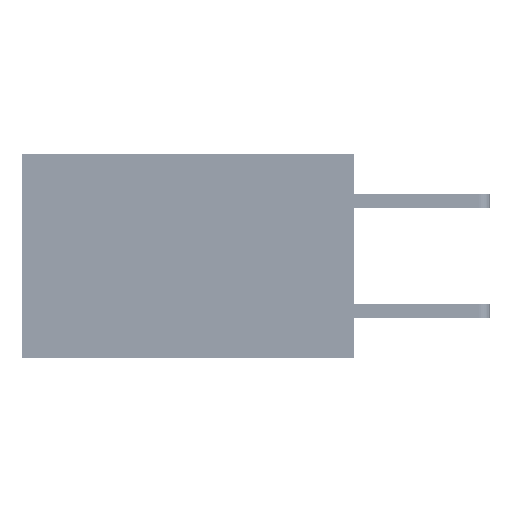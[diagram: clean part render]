
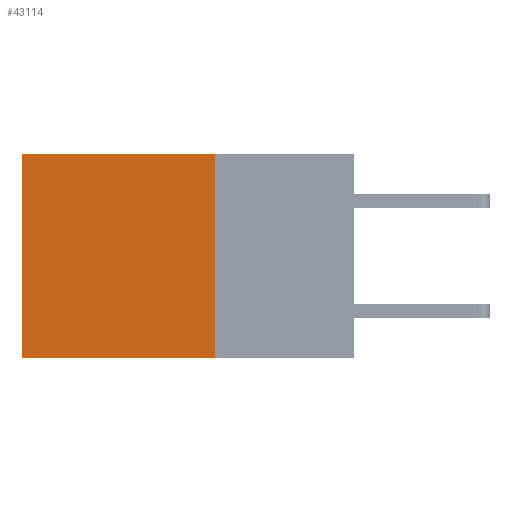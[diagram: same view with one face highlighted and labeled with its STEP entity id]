
A CAD part, left-side view. The second image highlights one B-rep face of the part: STEP entity #43114.
In plain terms, the highlighted planar face has unit normal (-1, 0, 0).
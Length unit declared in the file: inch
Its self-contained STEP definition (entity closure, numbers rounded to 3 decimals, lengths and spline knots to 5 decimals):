
#707 = DIRECTION ( 'NONE',  ( 0., 1., 0. ) ) ;
#711 = FACE_OUTER_BOUND ( 'NONE', #18224, .T. ) ;
#1418 = VERTEX_POINT ( 'NONE', #12976 ) ;
#2862 = LINE ( 'NONE', #3760, #28145 ) ;
#3760 = CARTESIAN_POINT ( 'NONE',  ( 0.2875, 0.6, 0. ) ) ;
#3798 = VERTEX_POINT ( 'NONE', #29327 ) ;
#6840 = LINE ( 'NONE', #11365, #21431 ) ;
#9747 = VECTOR ( 'NONE', #707, 39.37008 ) ;
#10970 = PLANE ( 'NONE',  #22107 ) ;
#11271 = DIRECTION ( 'NONE',  ( 0., 0., -1. ) ) ;
#11365 = CARTESIAN_POINT ( 'NONE',  ( 0.2875, 0.25, -0.37 ) ) ;
#12976 = CARTESIAN_POINT ( 'NONE',  ( 0.2875, 0.6, 0. ) ) ;
#13857 = CARTESIAN_POINT ( 'NONE',  ( 0.2875, 0.6, -0.37 ) ) ;
#14461 = CARTESIAN_POINT ( 'NONE',  ( 0.2875, 0.25, 0. ) ) ;
#14644 = LINE ( 'NONE', #18196, #9747 ) ;
#16017 = CARTESIAN_POINT ( 'NONE',  ( 0.2875, 0.25, 0. ) ) ;
#17931 = DIRECTION ( 'NONE',  ( 0., 0., -1. ) ) ;
#18196 = CARTESIAN_POINT ( 'NONE',  ( 0.2875, 0.25, 0. ) ) ;
#18224 = EDGE_LOOP ( 'NONE', ( #36121, #35545, #23854, #35601 ) ) ;
#20205 = LINE ( 'NONE', #16017, #27169 ) ;
#21431 = VECTOR ( 'NONE', #39453, 39.37008 ) ;
#22107 = AXIS2_PLACEMENT_3D ( 'NONE', #14461, #38490, #17931 ) ;
#23854 = ORIENTED_EDGE ( 'NONE', *, *, #33895, .F. ) ;
#27169 = VECTOR ( 'NONE', #36455, 39.37008 ) ;
#28145 = VECTOR ( 'NONE', #11271, 39.37008 ) ;
#29327 = CARTESIAN_POINT ( 'NONE',  ( 0.2875, 0.25, 0. ) ) ;
#29517 = VERTEX_POINT ( 'NONE', #37194 ) ;
#33895 = EDGE_CURVE ( 'NONE', #3798, #29517, #20205, .T. ) ;
#35545 = ORIENTED_EDGE ( 'NONE', *, *, #38626, .F. ) ;
#35601 = ORIENTED_EDGE ( 'NONE', *, *, #36529, .T. ) ;
#36121 = ORIENTED_EDGE ( 'NONE', *, *, #43061, .T. ) ;
#36455 = DIRECTION ( 'NONE',  ( 0., 0., -1. ) ) ;
#36529 = EDGE_CURVE ( 'NONE', #3798, #1418, #14644, .T. ) ;
#37194 = CARTESIAN_POINT ( 'NONE',  ( 0.2875, 0.25, -0.37 ) ) ;
#38490 = DIRECTION ( 'NONE',  ( 1., 0., 0. ) ) ;
#38626 = EDGE_CURVE ( 'NONE', #29517, #42971, #6840, .T. ) ;
#39453 = DIRECTION ( 'NONE',  ( 0., 1., 0. ) ) ;
#42971 = VERTEX_POINT ( 'NONE', #13857 ) ;
#43061 = EDGE_CURVE ( 'NONE', #1418, #42971, #2862, .T. ) ;
#43114 = ADVANCED_FACE ( 'NONE', ( #711 ), #10970, .F. ) ;
